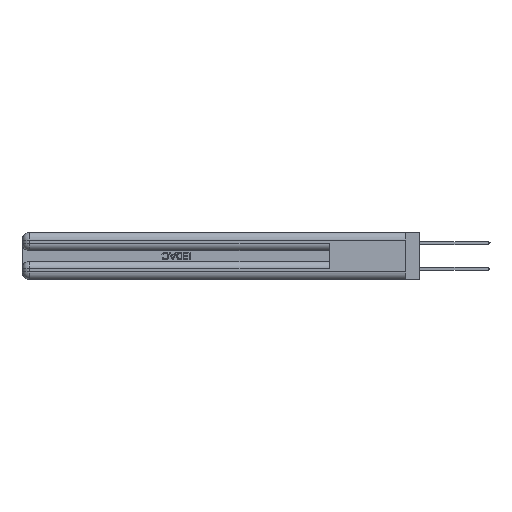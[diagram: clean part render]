
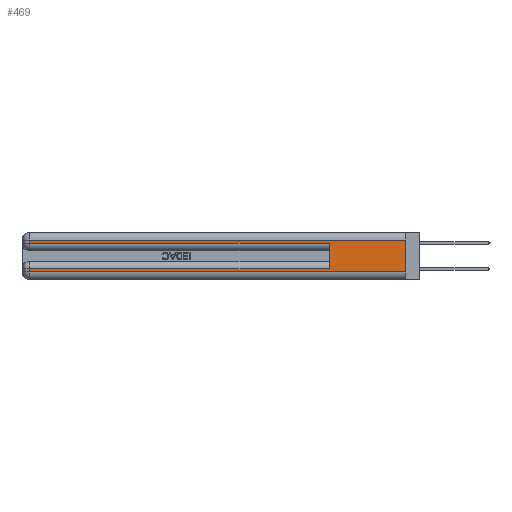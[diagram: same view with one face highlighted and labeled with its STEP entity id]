
A CAD part, left-side view. The second image highlights one B-rep face of the part: STEP entity #469.
In plain terms, the highlighted planar face has unit normal (-1, 0, 0).
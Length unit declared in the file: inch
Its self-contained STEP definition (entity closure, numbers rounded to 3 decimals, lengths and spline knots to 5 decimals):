
#114 = CARTESIAN_POINT ( 'NONE',  ( 0., 0., 0.085 ) ) ;
#347 = EDGE_CURVE ( 'NONE', #21355, #7710, #41753, .T. ) ;
#370 = ORIENTED_EDGE ( 'NONE', *, *, #9975, .T. ) ;
#469 = ADVANCED_FACE ( 'NONE', ( #32955 ), #44306, .F. ) ;
#2025 = DIRECTION ( 'NONE',  ( 0., 1., 0. ) ) ;
#2855 = EDGE_CURVE ( 'NONE', #29897, #38337, #43500, .T. ) ;
#3166 = DIRECTION ( 'NONE',  ( 1., 0., 0. ) ) ;
#3589 = DIRECTION ( 'NONE',  ( 0., -1., 0. ) ) ;
#3681 = LINE ( 'NONE', #45376, #24902 ) ;
#4208 = VECTOR ( 'NONE', #44152, 39.37008 ) ;
#6743 = CARTESIAN_POINT ( 'NONE',  ( 0., 0.6, 0.285 ) ) ;
#6796 = VERTEX_POINT ( 'NONE', #27280 ) ;
#7710 = VERTEX_POINT ( 'NONE', #37207 ) ;
#8434 = VECTOR ( 'NONE', #45493, 39.37008 ) ;
#8980 = LINE ( 'NONE', #114, #48423 ) ;
#9975 = EDGE_CURVE ( 'NONE', #38970, #6796, #8980, .T. ) ;
#10130 = LINE ( 'NONE', #32691, #4208 ) ;
#14056 = CARTESIAN_POINT ( 'NONE',  ( 0., 0.6, 0.085 ) ) ;
#15413 = VERTEX_POINT ( 'NONE', #28751 ) ;
#15436 = AXIS2_PLACEMENT_3D ( 'NONE', #18166, #3166, #22082 ) ;
#15930 = EDGE_CURVE ( 'NONE', #6796, #21355, #10130, .T. ) ;
#16296 = CARTESIAN_POINT ( 'NONE',  ( 0., 2.94, 0.06 ) ) ;
#16435 = VECTOR ( 'NONE', #2025, 39.37008 ) ;
#17318 = LINE ( 'NONE', #47232, #45527 ) ;
#18166 = CARTESIAN_POINT ( 'NONE',  ( 0., 0., 0.37 ) ) ;
#18758 = LINE ( 'NONE', #36014, #22289 ) ;
#19090 = ORIENTED_EDGE ( 'NONE', *, *, #24691, .F. ) ;
#21115 = CARTESIAN_POINT ( 'NONE',  ( 0., 2.94, 0.31 ) ) ;
#21355 = VERTEX_POINT ( 'NONE', #16296 ) ;
#22082 = DIRECTION ( 'NONE',  ( 0., 0., -1. ) ) ;
#22289 = VECTOR ( 'NONE', #43582, 39.37008 ) ;
#22611 = CARTESIAN_POINT ( 'NONE',  ( 0., 0., 0.31 ) ) ;
#22822 = DIRECTION ( 'NONE',  ( 0., 1., 0. ) ) ;
#22888 = VECTOR ( 'NONE', #45320, 39.37008 ) ;
#23981 = ORIENTED_EDGE ( 'NONE', *, *, #15930, .T. ) ;
#24691 = EDGE_CURVE ( 'NONE', #38970, #34851, #17318, .T. ) ;
#24902 = VECTOR ( 'NONE', #3589, 39.37008 ) ;
#24987 = EDGE_CURVE ( 'NONE', #15413, #34851, #3681, .T. ) ;
#25472 = EDGE_LOOP ( 'NONE', ( #25654, #36467, #40121, #29256, #19090, #370, #23981, #35805 ) ) ;
#25654 = ORIENTED_EDGE ( 'NONE', *, *, #25674, .F. ) ;
#25674 = EDGE_CURVE ( 'NONE', #29897, #7710, #33768, .T. ) ;
#27280 = CARTESIAN_POINT ( 'NONE',  ( 0., 2.94, 0.085 ) ) ;
#28751 = CARTESIAN_POINT ( 'NONE',  ( 0., 2.94, 0.285 ) ) ;
#29256 = ORIENTED_EDGE ( 'NONE', *, *, #24987, .T. ) ;
#29897 = VERTEX_POINT ( 'NONE', #22611 ) ;
#32691 = CARTESIAN_POINT ( 'NONE',  ( 0., 2.94, 0.37 ) ) ;
#32955 = FACE_OUTER_BOUND ( 'NONE', #25472, .T. ) ;
#33768 = LINE ( 'NONE', #37782, #8434 ) ;
#34020 = CARTESIAN_POINT ( 'NONE',  ( 0., 0., 0.06 ) ) ;
#34851 = VERTEX_POINT ( 'NONE', #6743 ) ;
#35305 = EDGE_CURVE ( 'NONE', #38337, #15413, #18758, .T. ) ;
#35805 = ORIENTED_EDGE ( 'NONE', *, *, #347, .T. ) ;
#36014 = CARTESIAN_POINT ( 'NONE',  ( 0., 2.94, 0.37 ) ) ;
#36467 = ORIENTED_EDGE ( 'NONE', *, *, #2855, .T. ) ;
#37207 = CARTESIAN_POINT ( 'NONE',  ( 0., 0., 0.06 ) ) ;
#37782 = CARTESIAN_POINT ( 'NONE',  ( 0., 0., 0.37 ) ) ;
#38337 = VERTEX_POINT ( 'NONE', #21115 ) ;
#38970 = VERTEX_POINT ( 'NONE', #14056 ) ;
#40121 = ORIENTED_EDGE ( 'NONE', *, *, #35305, .T. ) ;
#41753 = LINE ( 'NONE', #34020, #22888 ) ;
#43500 = LINE ( 'NONE', #46771, #16435 ) ;
#43582 = DIRECTION ( 'NONE',  ( 0., 0., -1. ) ) ;
#43632 = DIRECTION ( 'NONE',  ( 0., 0., 1. ) ) ;
#44152 = DIRECTION ( 'NONE',  ( 0., 0., -1. ) ) ;
#44306 = PLANE ( 'NONE',  #15436 ) ;
#45320 = DIRECTION ( 'NONE',  ( 0., -1., 0. ) ) ;
#45376 = CARTESIAN_POINT ( 'NONE',  ( 0., 0., 0.285 ) ) ;
#45493 = DIRECTION ( 'NONE',  ( 0., 0., -1. ) ) ;
#45527 = VECTOR ( 'NONE', #43632, 39.37008 ) ;
#46771 = CARTESIAN_POINT ( 'NONE',  ( 0., 0., 0.31 ) ) ;
#47232 = CARTESIAN_POINT ( 'NONE',  ( 0., 0.6, 0.145 ) ) ;
#48423 = VECTOR ( 'NONE', #22822, 39.37008 ) ;
